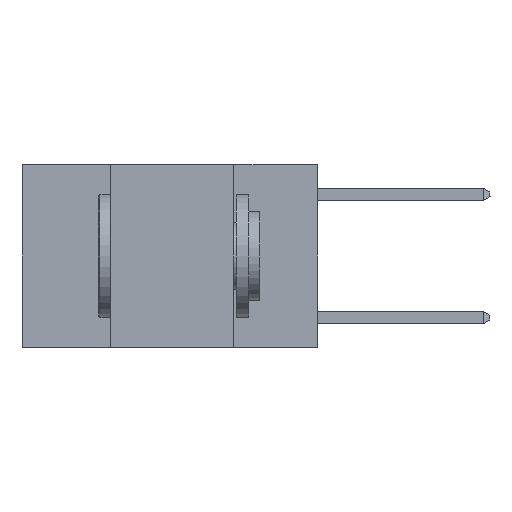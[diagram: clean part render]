
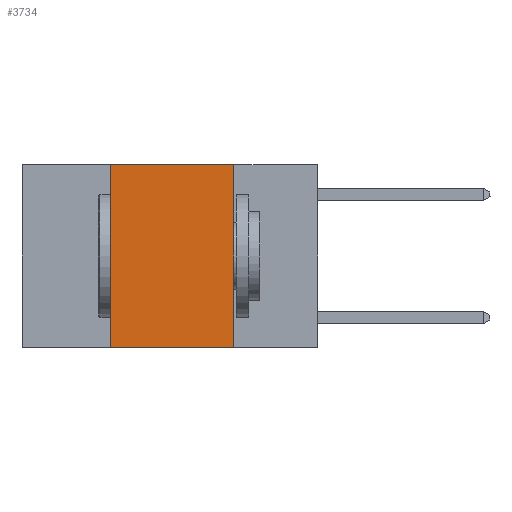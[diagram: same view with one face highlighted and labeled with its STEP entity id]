
A CAD part, left-side view. The second image highlights one B-rep face of the part: STEP entity #3734.
In plain terms, the highlighted planar face has unit normal (-1, 0, 0).
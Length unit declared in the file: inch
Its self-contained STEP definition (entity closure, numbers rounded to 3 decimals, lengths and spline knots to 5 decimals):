
#181 = LINE ( 'NONE', #7213, #198 ) ;
#198 = VECTOR ( 'NONE', #4771, 39.37008 ) ;
#411 = VERTEX_POINT ( 'NONE', #6478 ) ;
#659 = ORIENTED_EDGE ( 'NONE', *, *, #1100, .F. ) ;
#804 = PLANE ( 'NONE',  #8573 ) ;
#974 = ORIENTED_EDGE ( 'NONE', *, *, #3781, .T. ) ;
#1008 = ORIENTED_EDGE ( 'NONE', *, *, #1065, .F. ) ;
#1018 = ORIENTED_EDGE ( 'NONE', *, *, #6129, .F. ) ;
#1065 = EDGE_CURVE ( 'NONE', #7279, #3447, #7093, .T. ) ;
#1100 = EDGE_CURVE ( 'NONE', #411, #2260, #181, .T. ) ;
#2260 = VERTEX_POINT ( 'NONE', #5339 ) ;
#3417 = DIRECTION ( 'NONE',  ( 0., -1., 0. ) ) ;
#3447 = VERTEX_POINT ( 'NONE', #8445 ) ;
#3734 = ADVANCED_FACE ( 'NONE', ( #6305 ), #804, .F. ) ;
#3781 = EDGE_CURVE ( 'NONE', #7279, #2260, #5546, .T. ) ;
#4258 = EDGE_LOOP ( 'NONE', ( #659, #1018, #1008, #974 ) ) ;
#4512 = CARTESIAN_POINT ( 'NONE',  ( 0., 0.42, -0.37 ) ) ;
#4771 = DIRECTION ( 'NONE',  ( 0., 0., -1. ) ) ;
#4829 = VECTOR ( 'NONE', #7568, 39.37008 ) ;
#5037 = CARTESIAN_POINT ( 'NONE',  ( 0., 0.6, -0.37 ) ) ;
#5176 = CARTESIAN_POINT ( 'NONE',  ( 0., 0.6, 0. ) ) ;
#5339 = CARTESIAN_POINT ( 'NONE',  ( 0., 0.17, -0.37 ) ) ;
#5546 = LINE ( 'NONE', #5037, #4829 ) ;
#5623 = CARTESIAN_POINT ( 'NONE',  ( 0., 0.6, 0. ) ) ;
#5831 = VECTOR ( 'NONE', #3417, 39.37008 ) ;
#5841 = DIRECTION ( 'NONE',  ( 1., 0., 0. ) ) ;
#6129 = EDGE_CURVE ( 'NONE', #3447, #411, #7852, .T. ) ;
#6305 = FACE_OUTER_BOUND ( 'NONE', #4258, .T. ) ;
#6478 = CARTESIAN_POINT ( 'NONE',  ( 0., 0.17, 0. ) ) ;
#7071 = VECTOR ( 'NONE', #8078, 39.37008 ) ;
#7093 = LINE ( 'NONE', #8614, #7071 ) ;
#7213 = CARTESIAN_POINT ( 'NONE',  ( 0., 0.17, 0. ) ) ;
#7279 = VERTEX_POINT ( 'NONE', #4512 ) ;
#7568 = DIRECTION ( 'NONE',  ( 0., -1., 0. ) ) ;
#7852 = LINE ( 'NONE', #5176, #5831 ) ;
#7943 = DIRECTION ( 'NONE',  ( 0., 0., -1. ) ) ;
#8078 = DIRECTION ( 'NONE',  ( 0., 0., 1. ) ) ;
#8445 = CARTESIAN_POINT ( 'NONE',  ( 0., 0.42, 0. ) ) ;
#8573 = AXIS2_PLACEMENT_3D ( 'NONE', #5623, #5841, #7943 ) ;
#8614 = CARTESIAN_POINT ( 'NONE',  ( 0., 0.42, 0. ) ) ;
